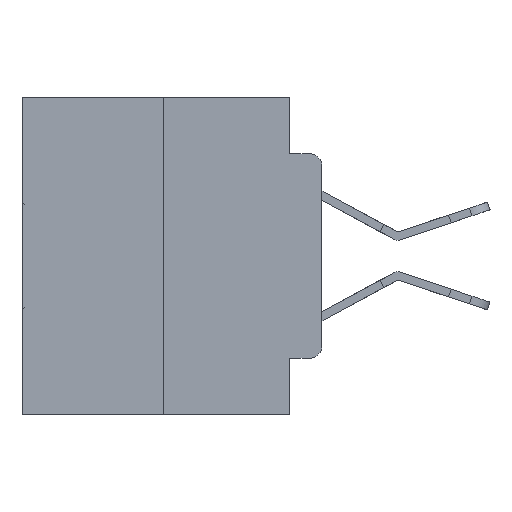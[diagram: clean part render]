
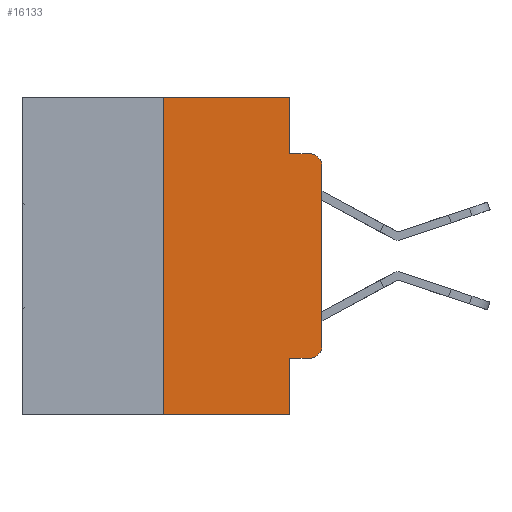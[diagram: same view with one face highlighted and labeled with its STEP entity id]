
A CAD part, left-side view. The second image highlights one B-rep face of the part: STEP entity #16133.
In plain terms, the highlighted planar face has unit normal (-1, 0, 0).
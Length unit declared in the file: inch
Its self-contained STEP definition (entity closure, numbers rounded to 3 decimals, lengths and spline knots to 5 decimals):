
#51 = LINE ( 'NONE', #3006, #21504 ) ;
#193 = EDGE_CURVE ( 'NONE', #6249, #14849, #14349, .T. ) ;
#1190 = VERTEX_POINT ( 'NONE', #16487 ) ;
#1291 = LINE ( 'NONE', #28717, #22398 ) ;
#1493 = CIRCLE ( 'NONE', #23532, 0.02 ) ;
#2417 = CARTESIAN_POINT ( 'NONE',  ( 0., 0.473, -0.5 ) ) ;
#2924 = CARTESIAN_POINT ( 'NONE',  ( 0., 0.25, 0. ) ) ;
#3006 = CARTESIAN_POINT ( 'NONE',  ( 0., 0.051, 0. ) ) ;
#3300 = EDGE_CURVE ( 'NONE', #5027, #16917, #6547, .T. ) ;
#3318 = CARTESIAN_POINT ( 'NONE',  ( 0., 0., 0. ) ) ;
#3657 = EDGE_CURVE ( 'NONE', #22296, #6249, #22055, .T. ) ;
#4972 = CARTESIAN_POINT ( 'NONE',  ( 0., 0.051, 0. ) ) ;
#5027 = VERTEX_POINT ( 'NONE', #5920 ) ;
#5411 = DIRECTION ( 'NONE',  ( -1., 0., 0. ) ) ;
#5668 = EDGE_CURVE ( 'NONE', #30158, #17934, #29374, .T. ) ;
#5920 = CARTESIAN_POINT ( 'NONE',  ( 0., 0.25, -0.5 ) ) ;
#5939 = VECTOR ( 'NONE', #17385, 39.37008 ) ;
#6112 = ORIENTED_EDGE ( 'NONE', *, *, #16582, .F. ) ;
#6249 = VERTEX_POINT ( 'NONE', #7130 ) ;
#6547 = LINE ( 'NONE', #2417, #12109 ) ;
#7130 = CARTESIAN_POINT ( 'NONE',  ( 0., 0., -0.1085 ) ) ;
#7638 = ORIENTED_EDGE ( 'NONE', *, *, #8973, .F. ) ;
#8332 = DIRECTION ( 'NONE',  ( 1., 0., 0. ) ) ;
#8933 = EDGE_CURVE ( 'NONE', #5027, #14504, #15868, .T. ) ;
#8967 = FACE_OUTER_BOUND ( 'NONE', #29555, .T. ) ;
#8973 = EDGE_CURVE ( 'NONE', #25291, #14849, #14036, .T. ) ;
#9300 = DIRECTION ( 'NONE',  ( 0., 0., -1. ) ) ;
#9570 = ORIENTED_EDGE ( 'NONE', *, *, #3300, .T. ) ;
#10196 = DIRECTION ( 'NONE',  ( 0., 0., -1. ) ) ;
#10282 = DIRECTION ( 'NONE',  ( 0., -1., 0. ) ) ;
#10484 = DIRECTION ( 'NONE',  ( 0., 0., 1. ) ) ;
#10878 = AXIS2_PLACEMENT_3D ( 'NONE', #20429, #8332, #20215 ) ;
#11271 = ORIENTED_EDGE ( 'NONE', *, *, #3657, .T. ) ;
#12109 = VECTOR ( 'NONE', #23728, 39.37008 ) ;
#12355 = CARTESIAN_POINT ( 'NONE',  ( 0., 0.02, -0.4115 ) ) ;
#12879 = ORIENTED_EDGE ( 'NONE', *, *, #8933, .F. ) ;
#13095 = ORIENTED_EDGE ( 'NONE', *, *, #20405, .F. ) ;
#14036 = LINE ( 'NONE', #24224, #16583 ) ;
#14349 = CIRCLE ( 'NONE', #24546, 0.02 ) ;
#14504 = VERTEX_POINT ( 'NONE', #21366 ) ;
#14551 = DIRECTION ( 'NONE',  ( 0., -1., 0. ) ) ;
#14849 = VERTEX_POINT ( 'NONE', #20527 ) ;
#15805 = VECTOR ( 'NONE', #10484, 39.37008 ) ;
#15868 = LINE ( 'NONE', #2924, #29929 ) ;
#16133 = ADVANCED_FACE ( 'NONE', ( #8967 ), #17738, .F. ) ;
#16487 = CARTESIAN_POINT ( 'NONE',  ( 0., 0.051, 0. ) ) ;
#16524 = EDGE_CURVE ( 'NONE', #1190, #25291, #51, .T. ) ;
#16582 = EDGE_CURVE ( 'NONE', #30158, #16917, #22613, .T. ) ;
#16583 = VECTOR ( 'NONE', #10282, 39.37008 ) ;
#16917 = VERTEX_POINT ( 'NONE', #18424 ) ;
#17385 = DIRECTION ( 'NONE',  ( 0., 0., -1. ) ) ;
#17738 = PLANE ( 'NONE',  #10878 ) ;
#17934 = VERTEX_POINT ( 'NONE', #12355 ) ;
#18424 = CARTESIAN_POINT ( 'NONE',  ( 0., 0.051, -0.5 ) ) ;
#19585 = CARTESIAN_POINT ( 'NONE',  ( 0., 0.02, -0.1085 ) ) ;
#20215 = DIRECTION ( 'NONE',  ( 0., 0., -1. ) ) ;
#20405 = EDGE_CURVE ( 'NONE', #14504, #1190, #1291, .T. ) ;
#20406 = CARTESIAN_POINT ( 'NONE',  ( 0., 0.051, -0.0885 ) ) ;
#20429 = CARTESIAN_POINT ( 'NONE',  ( 0., 0.473, 0. ) ) ;
#20527 = CARTESIAN_POINT ( 'NONE',  ( 0., 0.02, -0.0885 ) ) ;
#20673 = ORIENTED_EDGE ( 'NONE', *, *, #16524, .F. ) ;
#21035 = ORIENTED_EDGE ( 'NONE', *, *, #193, .T. ) ;
#21366 = CARTESIAN_POINT ( 'NONE',  ( 0., 0.25, 0. ) ) ;
#21504 = VECTOR ( 'NONE', #26676, 39.37008 ) ;
#21792 = CARTESIAN_POINT ( 'NONE',  ( 0., 0.051, -0.4115 ) ) ;
#22055 = LINE ( 'NONE', #3318, #15805 ) ;
#22296 = VERTEX_POINT ( 'NONE', #25464 ) ;
#22398 = VECTOR ( 'NONE', #14551, 39.37008 ) ;
#22613 = LINE ( 'NONE', #4972, #5939 ) ;
#22826 = ORIENTED_EDGE ( 'NONE', *, *, #25936, .T. ) ;
#23166 = CARTESIAN_POINT ( 'NONE',  ( 0., 0.02, -0.3915 ) ) ;
#23532 = AXIS2_PLACEMENT_3D ( 'NONE', #23166, #30415, #9300 ) ;
#23728 = DIRECTION ( 'NONE',  ( 0., -1., 0. ) ) ;
#24224 = CARTESIAN_POINT ( 'NONE',  ( 0., 0.051, -0.0885 ) ) ;
#24546 = AXIS2_PLACEMENT_3D ( 'NONE', #19585, #5411, #10196 ) ;
#25291 = VERTEX_POINT ( 'NONE', #20406 ) ;
#25464 = CARTESIAN_POINT ( 'NONE',  ( 0., 0., -0.3915 ) ) ;
#25476 = CARTESIAN_POINT ( 'NONE',  ( 0., 0.051, -0.4115 ) ) ;
#25936 = EDGE_CURVE ( 'NONE', #17934, #22296, #1493, .T. ) ;
#26040 = VECTOR ( 'NONE', #26384, 39.37008 ) ;
#26384 = DIRECTION ( 'NONE',  ( 0., -1., 0. ) ) ;
#26676 = DIRECTION ( 'NONE',  ( 0., 0., -1. ) ) ;
#28717 = CARTESIAN_POINT ( 'NONE',  ( 0., 0.473, 0. ) ) ;
#28984 = DIRECTION ( 'NONE',  ( 0., 0., 1. ) ) ;
#29374 = LINE ( 'NONE', #25476, #26040 ) ;
#29555 = EDGE_LOOP ( 'NONE', ( #11271, #21035, #7638, #20673, #13095, #12879, #9570, #6112, #30434, #22826 ) ) ;
#29929 = VECTOR ( 'NONE', #28984, 39.37008 ) ;
#30158 = VERTEX_POINT ( 'NONE', #21792 ) ;
#30415 = DIRECTION ( 'NONE',  ( -1., 0., 0. ) ) ;
#30434 = ORIENTED_EDGE ( 'NONE', *, *, #5668, .T. ) ;
